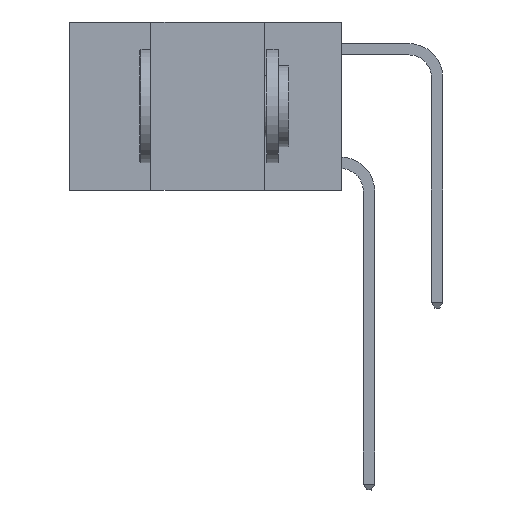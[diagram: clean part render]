
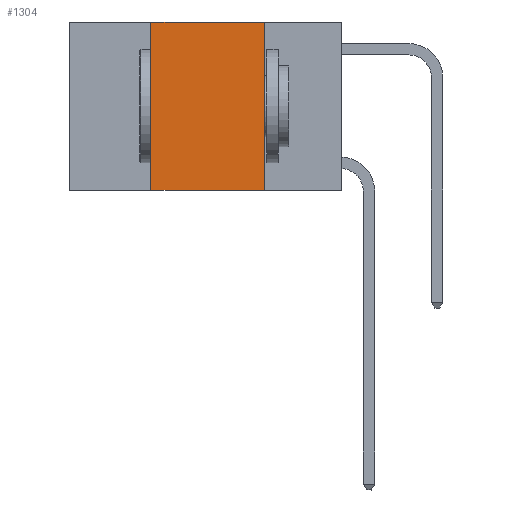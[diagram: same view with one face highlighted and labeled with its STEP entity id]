
A CAD part, left-side view. The second image highlights one B-rep face of the part: STEP entity #1304.
In plain terms, the highlighted planar face has unit normal (-1, 0, 0).
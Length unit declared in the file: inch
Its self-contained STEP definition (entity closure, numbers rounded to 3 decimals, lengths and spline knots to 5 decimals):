
#313 = CARTESIAN_POINT ( 'NONE',  ( 0., 0.6, 0. ) ) ;
#1026 = DIRECTION ( 'NONE',  ( 0., 0., -1. ) ) ;
#1039 = EDGE_CURVE ( 'NONE', #8758, #3982, #4218, .T. ) ;
#1050 = DIRECTION ( 'NONE',  ( 0., 0., -1. ) ) ;
#1147 = CARTESIAN_POINT ( 'NONE',  ( 0., 0.42, -0.37 ) ) ;
#1304 = ADVANCED_FACE ( 'NONE', ( #10948 ), #7599, .F. ) ;
#1753 = EDGE_CURVE ( 'NONE', #3982, #11195, #5313, .T. ) ;
#2238 = ORIENTED_EDGE ( 'NONE', *, *, #11617, .F. ) ;
#3440 = CARTESIAN_POINT ( 'NONE',  ( 0., 0.42, 0. ) ) ;
#3686 = CARTESIAN_POINT ( 'NONE',  ( 0., 0.17, -0.37 ) ) ;
#3982 = VERTEX_POINT ( 'NONE', #5476 ) ;
#4217 = CARTESIAN_POINT ( 'NONE',  ( 0., 0.6, 0. ) ) ;
#4218 = LINE ( 'NONE', #313, #11786 ) ;
#4610 = DIRECTION ( 'NONE',  ( 0., -1., 0. ) ) ;
#4664 = VECTOR ( 'NONE', #1026, 39.37008 ) ;
#4724 = ORIENTED_EDGE ( 'NONE', *, *, #1753, .F. ) ;
#4918 = EDGE_CURVE ( 'NONE', #12644, #11195, #11300, .T. ) ;
#5313 = LINE ( 'NONE', #10357, #4664 ) ;
#5476 = CARTESIAN_POINT ( 'NONE',  ( 0., 0.17, 0. ) ) ;
#6401 = AXIS2_PLACEMENT_3D ( 'NONE', #4217, #11194, #1050 ) ;
#7599 = PLANE ( 'NONE',  #6401 ) ;
#7611 = CARTESIAN_POINT ( 'NONE',  ( 0., 0.42, 0. ) ) ;
#8758 = VERTEX_POINT ( 'NONE', #7611 ) ;
#9191 = EDGE_LOOP ( 'NONE', ( #4724, #12926, #2238, #10498 ) ) ;
#9513 = DIRECTION ( 'NONE',  ( 0., -1., 0. ) ) ;
#10357 = CARTESIAN_POINT ( 'NONE',  ( 0., 0.17, 0. ) ) ;
#10498 = ORIENTED_EDGE ( 'NONE', *, *, #4918, .T. ) ;
#10652 = DIRECTION ( 'NONE',  ( 0., 0., 1. ) ) ;
#10709 = CARTESIAN_POINT ( 'NONE',  ( 0., 0.6, -0.37 ) ) ;
#10948 = FACE_OUTER_BOUND ( 'NONE', #9191, .T. ) ;
#10976 = VECTOR ( 'NONE', #4610, 39.37008 ) ;
#11194 = DIRECTION ( 'NONE',  ( 1., 0., 0. ) ) ;
#11195 = VERTEX_POINT ( 'NONE', #3686 ) ;
#11300 = LINE ( 'NONE', #10709, #10976 ) ;
#11617 = EDGE_CURVE ( 'NONE', #12644, #8758, #12066, .T. ) ;
#11786 = VECTOR ( 'NONE', #9513, 39.37008 ) ;
#12066 = LINE ( 'NONE', #3440, #12724 ) ;
#12644 = VERTEX_POINT ( 'NONE', #1147 ) ;
#12724 = VECTOR ( 'NONE', #10652, 39.37008 ) ;
#12926 = ORIENTED_EDGE ( 'NONE', *, *, #1039, .F. ) ;
